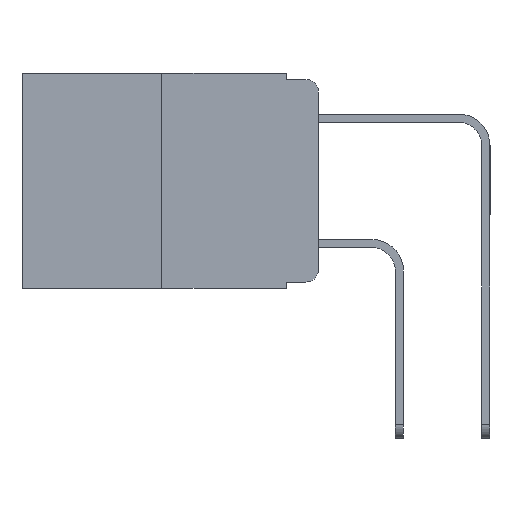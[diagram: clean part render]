
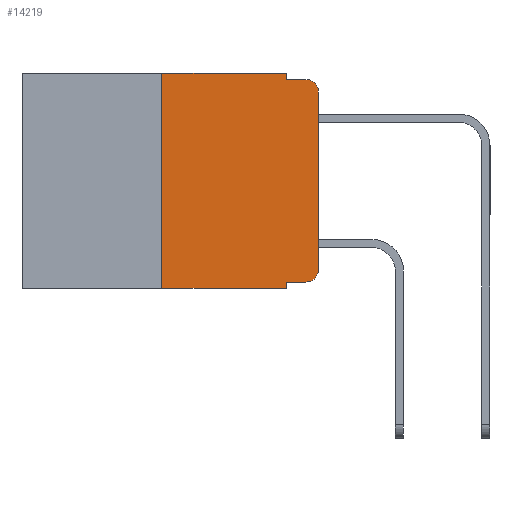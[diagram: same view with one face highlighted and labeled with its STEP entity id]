
A CAD part, left-side view. The second image highlights one B-rep face of the part: STEP entity #14219.
In plain terms, the highlighted planar face has unit normal (-1, 0, 0).
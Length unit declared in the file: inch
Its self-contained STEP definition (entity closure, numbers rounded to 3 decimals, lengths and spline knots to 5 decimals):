
#667 = PLANE ( 'NONE',  #16655 ) ;
#1237 = VERTEX_POINT ( 'NONE', #10977 ) ;
#1901 = LINE ( 'NONE', #15014, #6794 ) ;
#1996 = CARTESIAN_POINT ( 'NONE',  ( 0., 0.25, 0. ) ) ;
#3446 = ORIENTED_EDGE ( 'NONE', *, *, #11411, .T. ) ;
#3586 = VECTOR ( 'NONE', #3762, 39.37008 ) ;
#3682 = EDGE_CURVE ( 'NONE', #24395, #17808, #15256, .T. ) ;
#3762 = DIRECTION ( 'NONE',  ( 0., -1., 0. ) ) ;
#4086 = EDGE_CURVE ( 'NONE', #13647, #18739, #7420, .T. ) ;
#4265 = LINE ( 'NONE', #19769, #3586 ) ;
#4844 = DIRECTION ( 'NONE',  ( 0., 0., -1. ) ) ;
#4845 = VECTOR ( 'NONE', #13218, 39.37008 ) ;
#4975 = DIRECTION ( 'NONE',  ( 1., 0., 0. ) ) ;
#5471 = LINE ( 'NONE', #8957, #10251 ) ;
#5855 = EDGE_CURVE ( 'NONE', #14468, #1237, #20909, .T. ) ;
#6048 = AXIS2_PLACEMENT_3D ( 'NONE', #8362, #22119, #10401 ) ;
#6190 = DIRECTION ( 'NONE',  ( 0., 0., 1. ) ) ;
#6794 = VECTOR ( 'NONE', #7003, 39.37008 ) ;
#7003 = DIRECTION ( 'NONE',  ( 0., 0., 1. ) ) ;
#7078 = VERTEX_POINT ( 'NONE', #23995 ) ;
#7420 = CIRCLE ( 'NONE', #10468, 0.02 ) ;
#7508 = DIRECTION ( 'NONE',  ( -1., 0., 0. ) ) ;
#8362 = CARTESIAN_POINT ( 'NONE',  ( 0., 0.02, -0.313 ) ) ;
#8957 = CARTESIAN_POINT ( 'NONE',  ( 0., 0.051, 0. ) ) ;
#9257 = ORIENTED_EDGE ( 'NONE', *, *, #23599, .F. ) ;
#9776 = CARTESIAN_POINT ( 'NONE',  ( 0., 0.02, -0.333 ) ) ;
#9804 = CARTESIAN_POINT ( 'NONE',  ( 0., 0.25, -0.343 ) ) ;
#10251 = VECTOR ( 'NONE', #4844, 39.37008 ) ;
#10273 = LINE ( 'NONE', #18997, #4845 ) ;
#10401 = DIRECTION ( 'NONE',  ( 0., 0., -1. ) ) ;
#10468 = AXIS2_PLACEMENT_3D ( 'NONE', #19361, #7508, #21296 ) ;
#10977 = CARTESIAN_POINT ( 'NONE',  ( 0., 0., -0.313 ) ) ;
#11033 = CARTESIAN_POINT ( 'NONE',  ( 0., 0.051, 0. ) ) ;
#11290 = VERTEX_POINT ( 'NONE', #13395 ) ;
#11411 = EDGE_CURVE ( 'NONE', #12953, #14468, #20506, .T. ) ;
#11741 = DIRECTION ( 'NONE',  ( 0., -1., 0. ) ) ;
#12114 = FACE_OUTER_BOUND ( 'NONE', #25331, .T. ) ;
#12534 = VECTOR ( 'NONE', #16211, 39.37008 ) ;
#12686 = EDGE_CURVE ( 'NONE', #24395, #11290, #22845, .T. ) ;
#12749 = ORIENTED_EDGE ( 'NONE', *, *, #20549, .F. ) ;
#12953 = VERTEX_POINT ( 'NONE', #20843 ) ;
#12980 = EDGE_CURVE ( 'NONE', #17808, #22998, #10273, .T. ) ;
#13218 = DIRECTION ( 'NONE',  ( 0., -1., 0. ) ) ;
#13274 = CARTESIAN_POINT ( 'NONE',  ( 0., 0., -0.03 ) ) ;
#13361 = ORIENTED_EDGE ( 'NONE', *, *, #3682, .F. ) ;
#13395 = CARTESIAN_POINT ( 'NONE',  ( 0., 0.051, -0.343 ) ) ;
#13647 = VERTEX_POINT ( 'NONE', #13274 ) ;
#14219 = ADVANCED_FACE ( 'NONE', ( #12114 ), #667, .F. ) ;
#14446 = CARTESIAN_POINT ( 'NONE',  ( 0., 0.25, 0. ) ) ;
#14468 = VERTEX_POINT ( 'NONE', #9776 ) ;
#14891 = DIRECTION ( 'NONE',  ( 0., 0., -1. ) ) ;
#15014 = CARTESIAN_POINT ( 'NONE',  ( 0., 0., 0. ) ) ;
#15256 = LINE ( 'NONE', #1996, #25208 ) ;
#15587 = CARTESIAN_POINT ( 'NONE',  ( 0., 0.02, -0.01 ) ) ;
#16098 = VECTOR ( 'NONE', #14891, 39.37008 ) ;
#16211 = DIRECTION ( 'NONE',  ( 0., -1., 0. ) ) ;
#16655 = AXIS2_PLACEMENT_3D ( 'NONE', #16985, #4975, #18933 ) ;
#16677 = EDGE_CURVE ( 'NONE', #7078, #18739, #4265, .T. ) ;
#16985 = CARTESIAN_POINT ( 'NONE',  ( 0., 0.473, 0. ) ) ;
#17808 = VERTEX_POINT ( 'NONE', #14446 ) ;
#18198 = CARTESIAN_POINT ( 'NONE',  ( 0., 0.051, 0. ) ) ;
#18239 = ORIENTED_EDGE ( 'NONE', *, *, #12686, .T. ) ;
#18542 = EDGE_CURVE ( 'NONE', #1237, #13647, #1901, .T. ) ;
#18569 = ORIENTED_EDGE ( 'NONE', *, *, #4086, .T. ) ;
#18739 = VERTEX_POINT ( 'NONE', #15587 ) ;
#18933 = DIRECTION ( 'NONE',  ( 0., 0., -1. ) ) ;
#18997 = CARTESIAN_POINT ( 'NONE',  ( 0., 0.473, 0. ) ) ;
#19361 = CARTESIAN_POINT ( 'NONE',  ( 0., 0.02, -0.03 ) ) ;
#19769 = CARTESIAN_POINT ( 'NONE',  ( 0., 0.051, -0.01 ) ) ;
#20506 = LINE ( 'NONE', #25281, #24402 ) ;
#20549 = EDGE_CURVE ( 'NONE', #12953, #11290, #21239, .T. ) ;
#20843 = CARTESIAN_POINT ( 'NONE',  ( 0., 0.051, -0.333 ) ) ;
#20909 = CIRCLE ( 'NONE', #6048, 0.02 ) ;
#21239 = LINE ( 'NONE', #18198, #16098 ) ;
#21256 = ORIENTED_EDGE ( 'NONE', *, *, #16677, .F. ) ;
#21296 = DIRECTION ( 'NONE',  ( 0., 0., -1. ) ) ;
#22046 = CARTESIAN_POINT ( 'NONE',  ( 0., 0.473, -0.343 ) ) ;
#22119 = DIRECTION ( 'NONE',  ( -1., 0., 0. ) ) ;
#22845 = LINE ( 'NONE', #22046, #12534 ) ;
#22998 = VERTEX_POINT ( 'NONE', #11033 ) ;
#23599 = EDGE_CURVE ( 'NONE', #22998, #7078, #5471, .T. ) ;
#23995 = CARTESIAN_POINT ( 'NONE',  ( 0., 0.051, -0.01 ) ) ;
#24252 = ORIENTED_EDGE ( 'NONE', *, *, #12980, .F. ) ;
#24395 = VERTEX_POINT ( 'NONE', #9804 ) ;
#24402 = VECTOR ( 'NONE', #11741, 39.37008 ) ;
#24858 = ORIENTED_EDGE ( 'NONE', *, *, #18542, .T. ) ;
#24881 = ORIENTED_EDGE ( 'NONE', *, *, #5855, .T. ) ;
#25208 = VECTOR ( 'NONE', #6190, 39.37008 ) ;
#25281 = CARTESIAN_POINT ( 'NONE',  ( 0., 0.051, -0.333 ) ) ;
#25331 = EDGE_LOOP ( 'NONE', ( #24858, #18569, #21256, #9257, #24252, #13361, #18239, #12749, #3446, #24881 ) ) ;
